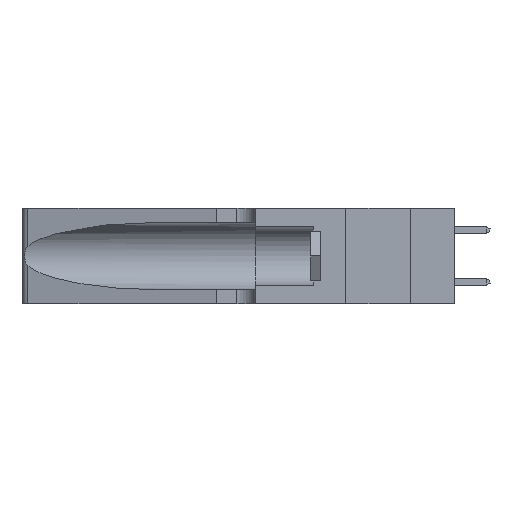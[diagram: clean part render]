
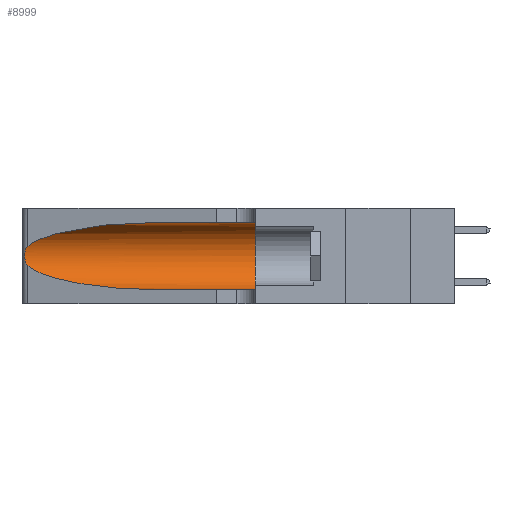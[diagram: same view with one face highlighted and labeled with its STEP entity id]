
A CAD part, left-side view. The second image highlights one B-rep face of the part: STEP entity #8999.
In plain terms, the highlighted cylindrical face has radius 3.308 mm (diameter 6.617 mm), a partial arc.
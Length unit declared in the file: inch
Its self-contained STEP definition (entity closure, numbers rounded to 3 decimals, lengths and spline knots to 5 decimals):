
#1047 = CARTESIAN_POINT ( 'NONE',  ( 0.2373, 1.15595, 0.28018 ) ) ;
#1834 = VECTOR ( 'NONE', #5210, 39.37008 ) ;
#2518 = CARTESIAN_POINT ( 'NONE',  ( 0.26017, 1.23833, 0.17102 ) ) ;
#2548 = EDGE_CURVE ( 'NONE', #13586, #13627, #19685, .T. ) ;
#2652 = CARTESIAN_POINT ( 'NONE',  ( 0.1305, 0.35, 0.31525 ) ) ;
#2781 = ORIENTED_EDGE ( 'NONE', *, *, #16688, .F. ) ;
#3475 = CARTESIAN_POINT ( 'NONE',  ( 0.1305, 0.72297, 0.31525 ) ) ;
#4342 = FACE_OUTER_BOUND ( 'NONE', #8372, .T. ) ;
#4385 = ORIENTED_EDGE ( 'NONE', *, *, #13099, .T. ) ;
#4630 = CARTESIAN_POINT ( 'NONE',  ( 0.1305, 1.61858, 0.05475 ) ) ;
#4761 = CARTESIAN_POINT ( 'NONE',  ( 0.1305, 1.61858, 0.185 ) ) ;
#5210 = DIRECTION ( 'NONE',  ( 0., -1., 0. ) ) ;
#5228 = VERTEX_POINT ( 'NONE', #19457 ) ;
#5469 = CARTESIAN_POINT ( 'NONE',  ( 0.25555, 1.22994, 0.2215 ) ) ;
#5604 = CARTESIAN_POINT ( 'NONE',  ( 0.25639, 1.23186, 0.15144 ) ) ;
#5606 = DIRECTION ( 'NONE',  ( 0., 1., 0. ) ) ;
#6049 = EDGE_CURVE ( 'NONE', #7238, #5228, #10598, .T. ) ;
#6551 = CYLINDRICAL_SURFACE ( 'NONE', #8501, 0.13025 ) ;
#7113 = CARTESIAN_POINT ( 'NONE',  ( 0.25555, 1.22993, 0.14849 ) ) ;
#7115 = CARTESIAN_POINT ( 'NONE',  ( 0.1305, 0.35, 0.185 ) ) ;
#7200 = CARTESIAN_POINT ( 'NONE',  ( 0.18966, 0.96281, 0.05475 ) ) ;
#7238 = VERTEX_POINT ( 'NONE', #19887 ) ;
#7990 = ORIENTED_EDGE ( 'NONE', *, *, #6049, .T. ) ;
#8372 = EDGE_LOOP ( 'NONE', ( #18100, #4385, #20072, #7990, #17186, #2781 ) ) ;
#8434 = B_SPLINE_CURVE_WITH_KNOTS ( 'NONE', 3,
 ( #9928, #5469, #11888, #10401, #18318, #10465, #19602, #16490, #2518, #13472, #15191, #5604, #7113, #15059 ),
 .UNSPECIFIED., .F., .F.,
 ( 4, 2, 2, 2, 2, 2, 4 ),
 ( 0., 0.00027, 0.00053, 0.00107, 0.0016, 0.00187, 0.00214 ),
 .UNSPECIFIED. ) ;
#8501 = AXIS2_PLACEMENT_3D ( 'NONE', #4761, #18722, #15729 ) ;
#8999 = ADVANCED_FACE ( 'NONE', ( #4342 ), #6551, .F. ) ;
#9222 = DIRECTION ( 'NONE',  ( 0., -1., 0. ) ) ;
#9928 = CARTESIAN_POINT ( 'NONE',  ( 0.25487, 1.22718, 0.22369 ) ) ;
#10401 = CARTESIAN_POINT ( 'NONE',  ( 0.25787, 1.23484, 0.2124 ) ) ;
#10451 = CARTESIAN_POINT ( 'NONE',  ( 0.18966, 0.96281, 0.31525 ) ) ;
#10465 = CARTESIAN_POINT ( 'NONE',  ( 0.26018, 1.23835, 0.19895 ) ) ;
#10598 = LINE ( 'NONE', #4630, #16729 ) ;
#10845 = AXIS2_PLACEMENT_3D ( 'NONE', #7115, #5606, #17917 ) ;
#11329 = VERTEX_POINT ( 'NONE', #11881 ) ;
#11881 = CARTESIAN_POINT ( 'NONE',  ( 0.25487, 1.22718, 0.14631 ) ) ;
#11888 = CARTESIAN_POINT ( 'NONE',  ( 0.25639, 1.23184, 0.21858 ) ) ;
#12004 = CARTESIAN_POINT ( 'NONE',  ( 0.25487, 1.22718, 0.22369 ) ) ;
#13099 = EDGE_CURVE ( 'NONE', #13627, #11329, #8434, .T. ) ;
#13371 = CARTESIAN_POINT ( 'NONE',  ( 0.25487, 1.22718, 0.22369 ) ) ;
#13472 = CARTESIAN_POINT ( 'NONE',  ( 0.25856, 1.23593, 0.16098 ) ) ;
#13586 = VERTEX_POINT ( 'NONE', #3475 ) ;
#13627 = VERTEX_POINT ( 'NONE', #13371 ) ;
#13861 = CARTESIAN_POINT ( 'NONE',  ( 0.1305, 0.72297, 0.31525 ) ) ;
#14194 =( BOUNDED_CURVE ( )  B_SPLINE_CURVE ( 3, ( #16499, #18064, #7200, #19615 ),
 .UNSPECIFIED., .F., .F. ) 
 B_SPLINE_CURVE_WITH_KNOTS ( ( 4, 4 ),
 ( 3.44316, 4.71239 ),
 .UNSPECIFIED. ) 
 CURVE ( )  GEOMETRIC_REPRESENTATION_ITEM ( )  RATIONAL_B_SPLINE_CURVE ( ( 1., 0.87, 0.87, 1. ) ) 
 REPRESENTATION_ITEM ( '' )  );
#15059 = CARTESIAN_POINT ( 'NONE',  ( 0.25487, 1.22718, 0.14631 ) ) ;
#15191 = CARTESIAN_POINT ( 'NONE',  ( 0.25789, 1.23486, 0.15765 ) ) ;
#15729 = DIRECTION ( 'NONE',  ( 0., 0., -1. ) ) ;
#16349 = EDGE_CURVE ( 'NONE', #16525, #5228, #18021, .T. ) ;
#16490 = CARTESIAN_POINT ( 'NONE',  ( 0.26075, 1.23896, 0.178 ) ) ;
#16499 = CARTESIAN_POINT ( 'NONE',  ( 0.25487, 1.22718, 0.14631 ) ) ;
#16525 = VERTEX_POINT ( 'NONE', #2652 ) ;
#16688 = EDGE_CURVE ( 'NONE', #13586, #16525, #17762, .T. ) ;
#16729 = VECTOR ( 'NONE', #9222, 39.37008 ) ;
#17186 = ORIENTED_EDGE ( 'NONE', *, *, #16349, .F. ) ;
#17762 = LINE ( 'NONE', #20167, #1834 ) ;
#17917 = DIRECTION ( 'NONE',  ( 0., 0., 1. ) ) ;
#18021 = CIRCLE ( 'NONE', #10845, 0.13025 ) ;
#18064 = CARTESIAN_POINT ( 'NONE',  ( 0.2373, 1.15595, 0.08982 ) ) ;
#18100 = ORIENTED_EDGE ( 'NONE', *, *, #2548, .T. ) ;
#18318 = CARTESIAN_POINT ( 'NONE',  ( 0.25854, 1.2359, 0.20912 ) ) ;
#18722 = DIRECTION ( 'NONE',  ( 0., -1., 0. ) ) ;
#18818 = EDGE_CURVE ( 'NONE', #11329, #7238, #14194, .T. ) ;
#19457 = CARTESIAN_POINT ( 'NONE',  ( 0.1305, 0.35, 0.05475 ) ) ;
#19602 = CARTESIAN_POINT ( 'NONE',  ( 0.26075, 1.23896, 0.19203 ) ) ;
#19615 = CARTESIAN_POINT ( 'NONE',  ( 0.1305, 0.72297, 0.05475 ) ) ;
#19685 =( BOUNDED_CURVE ( )  B_SPLINE_CURVE ( 3, ( #13861, #10451, #1047, #12004 ),
 .UNSPECIFIED., .F., .T. ) 
 B_SPLINE_CURVE_WITH_KNOTS ( ( 4, 4 ),
 ( 1.5708, 2.84003 ),
 .UNSPECIFIED. ) 
 CURVE ( )  GEOMETRIC_REPRESENTATION_ITEM ( )  RATIONAL_B_SPLINE_CURVE ( ( 1., 0.87, 0.87, 1. ) ) 
 REPRESENTATION_ITEM ( '' )  );
#19887 = CARTESIAN_POINT ( 'NONE',  ( 0.1305, 0.72297, 0.05475 ) ) ;
#20072 = ORIENTED_EDGE ( 'NONE', *, *, #18818, .T. ) ;
#20167 = CARTESIAN_POINT ( 'NONE',  ( 0.1305, 1.61858, 0.31525 ) ) ;
